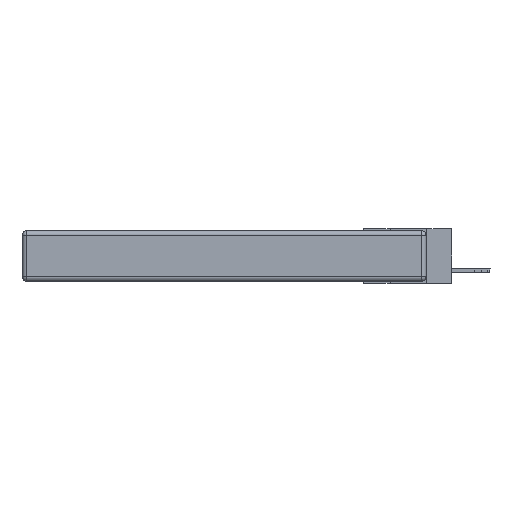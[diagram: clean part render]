
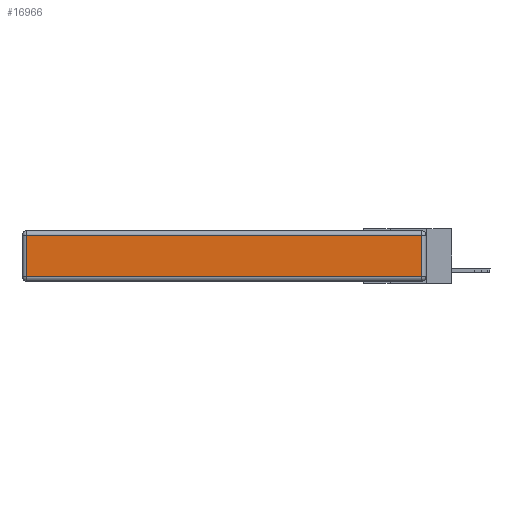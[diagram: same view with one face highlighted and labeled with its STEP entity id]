
A CAD part, left-side view. The second image highlights one B-rep face of the part: STEP entity #16966.
In plain terms, the highlighted planar face has unit normal (-1, 0, 0).
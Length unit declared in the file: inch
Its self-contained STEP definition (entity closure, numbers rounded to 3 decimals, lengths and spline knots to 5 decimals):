
#120 = LINE ( 'NONE', #10020, #16443 ) ;
#254 = VECTOR ( 'NONE', #8426, 39.37008 ) ;
#771 = CARTESIAN_POINT ( 'NONE',  ( 0., 2.72, -0.03 ) ) ;
#925 = VERTEX_POINT ( 'NONE', #18604 ) ;
#1084 = LINE ( 'NONE', #19230, #15719 ) ;
#1162 = PLANE ( 'NONE',  #10559 ) ;
#1793 = VECTOR ( 'NONE', #16669, 39.37008 ) ;
#1853 = EDGE_LOOP ( 'NONE', ( #8936, #6243, #8722, #10407 ) ) ;
#1895 = LINE ( 'NONE', #15907, #254 ) ;
#2484 = LINE ( 'NONE', #10543, #1793 ) ;
#4428 = VERTEX_POINT ( 'NONE', #12685 ) ;
#4800 = DIRECTION ( 'NONE',  ( 0., 0., -1. ) ) ;
#5002 = EDGE_CURVE ( 'NONE', #12613, #925, #2484, .T. ) ;
#5552 = DIRECTION ( 'NONE',  ( 0., 1., 0. ) ) ;
#6243 = ORIENTED_EDGE ( 'NONE', *, *, #5002, .T. ) ;
#6741 = VERTEX_POINT ( 'NONE', #771 ) ;
#8426 = DIRECTION ( 'NONE',  ( 0., -1., 0. ) ) ;
#8722 = ORIENTED_EDGE ( 'NONE', *, *, #18433, .T. ) ;
#8936 = ORIENTED_EDGE ( 'NONE', *, *, #15429, .T. ) ;
#10020 = CARTESIAN_POINT ( 'NONE',  ( 0., 2.75, -0.03 ) ) ;
#10407 = ORIENTED_EDGE ( 'NONE', *, *, #13107, .T. ) ;
#10543 = CARTESIAN_POINT ( 'NONE',  ( 0., 0.03, -0.343 ) ) ;
#10559 = AXIS2_PLACEMENT_3D ( 'NONE', #13050, #17555, #14488 ) ;
#12242 = CARTESIAN_POINT ( 'NONE',  ( 0., 0.03, -0.313 ) ) ;
#12613 = VERTEX_POINT ( 'NONE', #12242 ) ;
#12685 = CARTESIAN_POINT ( 'NONE',  ( 0., 2.72, -0.313 ) ) ;
#13050 = CARTESIAN_POINT ( 'NONE',  ( 0., 0., -0.343 ) ) ;
#13107 = EDGE_CURVE ( 'NONE', #6741, #4428, #1084, .T. ) ;
#14488 = DIRECTION ( 'NONE',  ( 0., 0., 1. ) ) ;
#15429 = EDGE_CURVE ( 'NONE', #4428, #12613, #1895, .T. ) ;
#15719 = VECTOR ( 'NONE', #4800, 39.37008 ) ;
#15907 = CARTESIAN_POINT ( 'NONE',  ( 0., 0., -0.313 ) ) ;
#16443 = VECTOR ( 'NONE', #5552, 39.37008 ) ;
#16502 = FACE_OUTER_BOUND ( 'NONE', #1853, .T. ) ;
#16669 = DIRECTION ( 'NONE',  ( 0., 0., 1. ) ) ;
#16966 = ADVANCED_FACE ( 'NONE', ( #16502 ), #1162, .T. ) ;
#17555 = DIRECTION ( 'NONE',  ( -1., 0., 0. ) ) ;
#18433 = EDGE_CURVE ( 'NONE', #925, #6741, #120, .T. ) ;
#18604 = CARTESIAN_POINT ( 'NONE',  ( 0., 0.03, -0.03 ) ) ;
#19230 = CARTESIAN_POINT ( 'NONE',  ( 0., 2.72, -0.343 ) ) ;
